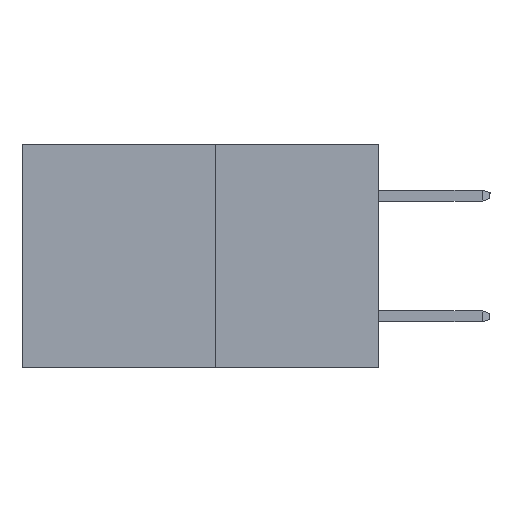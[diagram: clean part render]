
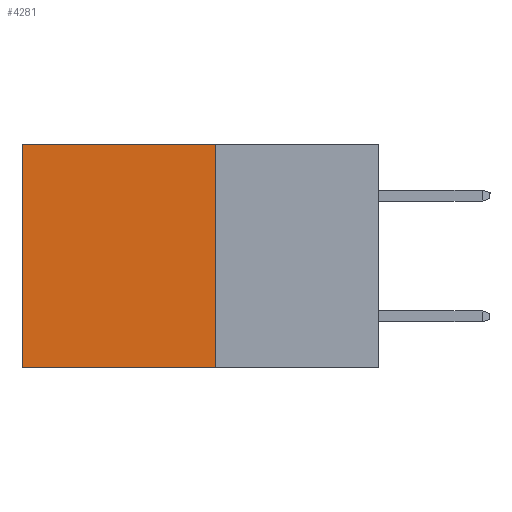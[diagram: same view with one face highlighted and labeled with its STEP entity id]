
A CAD part, left-side view. The second image highlights one B-rep face of the part: STEP entity #4281.
In plain terms, the highlighted planar face has unit normal (-1, 0, 0).
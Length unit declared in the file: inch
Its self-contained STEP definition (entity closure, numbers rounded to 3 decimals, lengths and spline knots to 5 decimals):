
#609 = ORIENTED_EDGE ( 'NONE', *, *, #5224, .T. ) ;
#915 = CARTESIAN_POINT ( 'NONE',  ( 0.277, 0.27, 0. ) ) ;
#1444 = CARTESIAN_POINT ( 'NONE',  ( 0.277, 0.59, -0.37 ) ) ;
#2205 = EDGE_CURVE ( 'NONE', #3117, #3880, #4035, .T. ) ;
#2416 = EDGE_CURVE ( 'NONE', #8012, #3214, #4355, .T. ) ;
#2499 = ORIENTED_EDGE ( 'NONE', *, *, #2641, .F. ) ;
#2555 = VECTOR ( 'NONE', #4636, 39.37008 ) ;
#2641 = EDGE_CURVE ( 'NONE', #3880, #3214, #2886, .T. ) ;
#2872 = EDGE_LOOP ( 'NONE', ( #7654, #2499, #2901, #609 ) ) ;
#2886 = LINE ( 'NONE', #3931, #7831 ) ;
#2901 = ORIENTED_EDGE ( 'NONE', *, *, #2205, .F. ) ;
#3117 = VERTEX_POINT ( 'NONE', #915 ) ;
#3214 = VERTEX_POINT ( 'NONE', #4466 ) ;
#3289 = CARTESIAN_POINT ( 'NONE',  ( 0.277, 0.27, -0.37 ) ) ;
#3880 = VERTEX_POINT ( 'NONE', #3289 ) ;
#3931 = CARTESIAN_POINT ( 'NONE',  ( 0.277, 0.27, -0.37 ) ) ;
#3990 = VECTOR ( 'NONE', #6703, 39.37008 ) ;
#4035 = LINE ( 'NONE', #6160, #7287 ) ;
#4206 = LINE ( 'NONE', #4526, #3990 ) ;
#4281 = ADVANCED_FACE ( 'NONE', ( #8378 ), #5096, .F. ) ;
#4355 = LINE ( 'NONE', #1444, #2555 ) ;
#4466 = CARTESIAN_POINT ( 'NONE',  ( 0.277, 0.59, -0.37 ) ) ;
#4526 = CARTESIAN_POINT ( 'NONE',  ( 0.277, 0.27, 0. ) ) ;
#4636 = DIRECTION ( 'NONE',  ( 0., 0., -1. ) ) ;
#4892 = CARTESIAN_POINT ( 'NONE',  ( 0.277, 0.27, -0.37 ) ) ;
#5096 = PLANE ( 'NONE',  #5798 ) ;
#5224 = EDGE_CURVE ( 'NONE', #3117, #8012, #4206, .T. ) ;
#5236 = DIRECTION ( 'NONE',  ( 0., 0., -1. ) ) ;
#5798 = AXIS2_PLACEMENT_3D ( 'NONE', #4892, #7550, #5236 ) ;
#6160 = CARTESIAN_POINT ( 'NONE',  ( 0.277, 0.27, -0.37 ) ) ;
#6703 = DIRECTION ( 'NONE',  ( 0., 1., 0. ) ) ;
#6778 = DIRECTION ( 'NONE',  ( 0., 1., 0. ) ) ;
#7287 = VECTOR ( 'NONE', #8217, 39.37008 ) ;
#7459 = CARTESIAN_POINT ( 'NONE',  ( 0.277, 0.59, 0. ) ) ;
#7550 = DIRECTION ( 'NONE',  ( 1., 0., 0. ) ) ;
#7654 = ORIENTED_EDGE ( 'NONE', *, *, #2416, .T. ) ;
#7831 = VECTOR ( 'NONE', #6778, 39.37008 ) ;
#8012 = VERTEX_POINT ( 'NONE', #7459 ) ;
#8217 = DIRECTION ( 'NONE',  ( 0., 0., -1. ) ) ;
#8378 = FACE_OUTER_BOUND ( 'NONE', #2872, .T. ) ;
